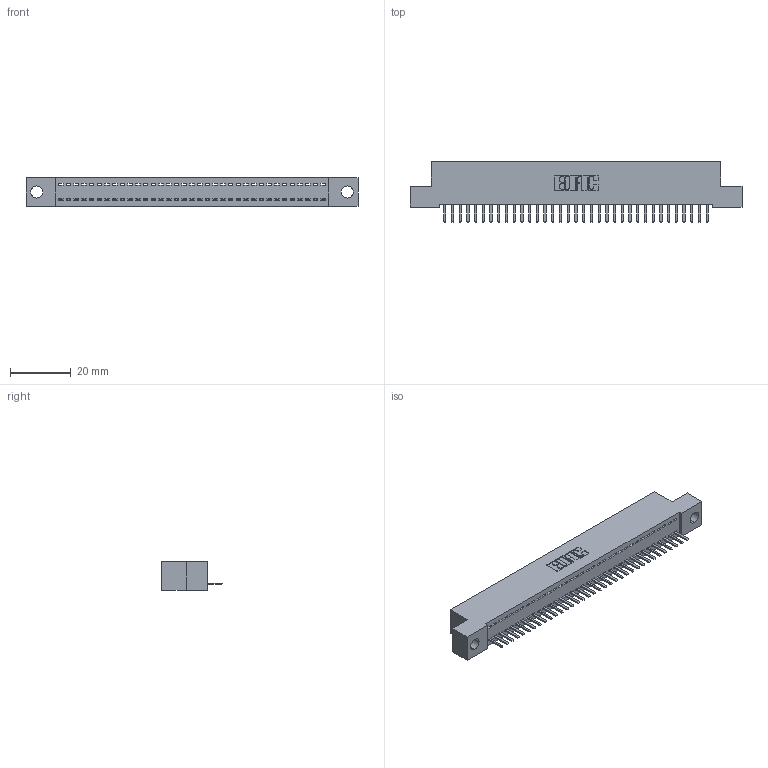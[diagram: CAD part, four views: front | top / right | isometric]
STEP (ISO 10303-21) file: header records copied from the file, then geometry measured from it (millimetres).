
FILE_DESCRIPTION (( 'STEP AP203' ), '1' );
FILE_NAME ('342-035-520-104.STEP', '2018-08-11T19:15:46', ( '' ), ( '' ), 'SwSTEP 2.0', 'SolidWorks 2016', '' );
FILE_SCHEMA (( 'CONFIG_CONTROL_DESIGN' ));
Length unit declared in the file: inch
Products named in the file (3): 342 Part_.156 TH; 345-292-001_345-293-120; 342-035-520-104
Assembly tree (36 placements, depth 2):
  342-035-520-104
    342 Part_.156 TH
    345-292-001_345-293-120  x35
Bounding box: 109.22 x 20.02 x 9.4 mm (x, y, z)
Volume: 9362.9 mm3; surface area: 13115.1 mm2
Topology: 36 solids, 36 shells, 2280 faces, 6739 edges, 4398 vertices
Faces by surface type: plane 1606, cylinder 674
Entity records: 22287 total; most frequent: CARTESIAN_POINT 3863, ORIENTED_EDGE 3822, DIRECTION 3261, EDGE_CURVE 1911, VECTOR 1779, LINE 1779, VERTEX_POINT 1270, AXIS2_PLACEMENT_3D 741
